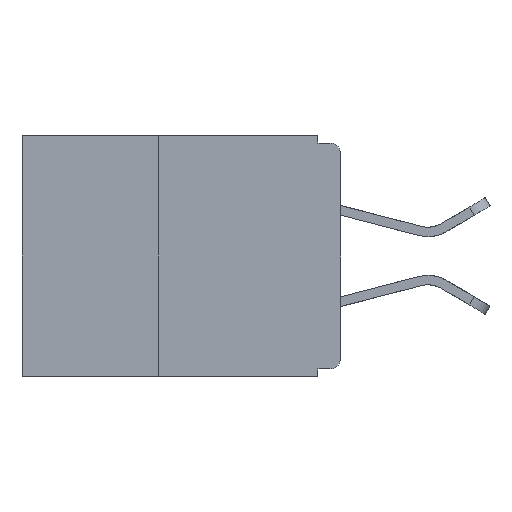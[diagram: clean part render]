
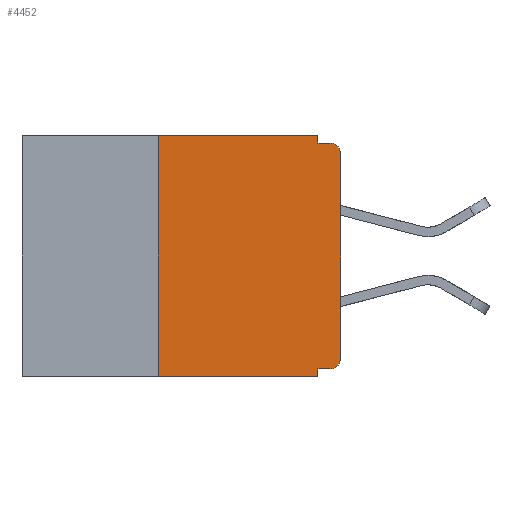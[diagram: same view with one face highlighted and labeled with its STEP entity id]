
A CAD part, left-side view. The second image highlights one B-rep face of the part: STEP entity #4452.
In plain terms, the highlighted planar face has unit normal (-1, 0, 0).
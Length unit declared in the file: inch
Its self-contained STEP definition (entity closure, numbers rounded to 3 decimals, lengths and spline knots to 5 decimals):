
#383 = DIRECTION ( 'NONE',  ( 1., 0., 0. ) ) ;
#982 = VECTOR ( 'NONE', #26300, 39.37008 ) ;
#1465 = CARTESIAN_POINT ( 'NONE',  ( 0., 0.437, 0. ) ) ;
#1678 = DIRECTION ( 'NONE',  ( 0., -1., 0. ) ) ;
#1950 = EDGE_CURVE ( 'NONE', #2396, #4100, #3413, .T. ) ;
#2301 = AXIS2_PLACEMENT_3D ( 'NONE', #21754, #9430, #23759 ) ;
#2396 = VERTEX_POINT ( 'NONE', #19117 ) ;
#2448 = CARTESIAN_POINT ( 'NONE',  ( 0., 0., -0.305 ) ) ;
#2530 = EDGE_CURVE ( 'NONE', #22444, #8970, #4804, .T. ) ;
#2553 = VERTEX_POINT ( 'NONE', #17504 ) ;
#2734 = CIRCLE ( 'NONE', #2301, 0.015 ) ;
#3050 = LINE ( 'NONE', #20234, #24468 ) ;
#3413 = CIRCLE ( 'NONE', #8752, 0.015 ) ;
#3708 = CARTESIAN_POINT ( 'NONE',  ( 0., 0.031, 0. ) ) ;
#3737 = PLANE ( 'NONE',  #25244 ) ;
#4100 = VERTEX_POINT ( 'NONE', #2448 ) ;
#4102 = LINE ( 'NONE', #18212, #24798 ) ;
#4452 = ADVANCED_FACE ( 'NONE', ( #10992 ), #3737, .F. ) ;
#4738 = VERTEX_POINT ( 'NONE', #19252 ) ;
#4804 = LINE ( 'NONE', #23291, #26603 ) ;
#5505 = LINE ( 'NONE', #3708, #982 ) ;
#6518 = EDGE_LOOP ( 'NONE', ( #24944, #15707, #7336, #26795, #16690, #24692, #26498, #8674, #20303, #11308 ) ) ;
#7336 = ORIENTED_EDGE ( 'NONE', *, *, #2530, .F. ) ;
#8523 = DIRECTION ( 'NONE',  ( 0., -1., 0. ) ) ;
#8674 = ORIENTED_EDGE ( 'NONE', *, *, #22145, .F. ) ;
#8752 = AXIS2_PLACEMENT_3D ( 'NONE', #15253, #18002, #26959 ) ;
#8970 = VERTEX_POINT ( 'NONE', #23158 ) ;
#9430 = DIRECTION ( 'NONE',  ( -1., 0., 0. ) ) ;
#10110 = DIRECTION ( 'NONE',  ( 0., 0., 1. ) ) ;
#10992 = FACE_OUTER_BOUND ( 'NONE', #6518, .T. ) ;
#11157 = EDGE_CURVE ( 'NONE', #4738, #22444, #5505, .T. ) ;
#11308 = ORIENTED_EDGE ( 'NONE', *, *, #1950, .T. ) ;
#11606 = LINE ( 'NONE', #24919, #21892 ) ;
#11624 = EDGE_CURVE ( 'NONE', #4100, #22159, #4102, .T. ) ;
#12183 = DIRECTION ( 'NONE',  ( 0., 1., 0. ) ) ;
#12957 = CARTESIAN_POINT ( 'NONE',  ( 0., 0.437, 0. ) ) ;
#14311 = CARTESIAN_POINT ( 'NONE',  ( 0., 0.25, 0. ) ) ;
#14985 = DIRECTION ( 'NONE',  ( 0., -1., 0. ) ) ;
#15226 = CARTESIAN_POINT ( 'NONE',  ( 0., 0.031, -0.01 ) ) ;
#15237 = EDGE_CURVE ( 'NONE', #19847, #19323, #3050, .T. ) ;
#15253 = CARTESIAN_POINT ( 'NONE',  ( 0., 0.015, -0.305 ) ) ;
#15657 = LINE ( 'NONE', #24407, #22442 ) ;
#15707 = ORIENTED_EDGE ( 'NONE', *, *, #24796, .T. ) ;
#16602 = EDGE_CURVE ( 'NONE', #19847, #25715, #11606, .T. ) ;
#16690 = ORIENTED_EDGE ( 'NONE', *, *, #21731, .F. ) ;
#17324 = LINE ( 'NONE', #12957, #22165 ) ;
#17504 = CARTESIAN_POINT ( 'NONE',  ( 0., 0.031, -0.32 ) ) ;
#17932 = EDGE_CURVE ( 'NONE', #2396, #2553, #15657, .T. ) ;
#18002 = DIRECTION ( 'NONE',  ( -1., 0., 0. ) ) ;
#18177 = DIRECTION ( 'NONE',  ( 0., 0., 1. ) ) ;
#18212 = CARTESIAN_POINT ( 'NONE',  ( 0., 0., 0. ) ) ;
#19117 = CARTESIAN_POINT ( 'NONE',  ( 0., 0.015, -0.32 ) ) ;
#19252 = CARTESIAN_POINT ( 'NONE',  ( 0., 0.031, 0. ) ) ;
#19323 = VERTEX_POINT ( 'NONE', #14311 ) ;
#19847 = VERTEX_POINT ( 'NONE', #26520 ) ;
#20234 = CARTESIAN_POINT ( 'NONE',  ( 0., 0.25, -0.33 ) ) ;
#20303 = ORIENTED_EDGE ( 'NONE', *, *, #17932, .F. ) ;
#20421 = CARTESIAN_POINT ( 'NONE',  ( 0., 0., -0.025 ) ) ;
#21528 = VECTOR ( 'NONE', #22455, 39.37008 ) ;
#21731 = EDGE_CURVE ( 'NONE', #19323, #4738, #17324, .T. ) ;
#21754 = CARTESIAN_POINT ( 'NONE',  ( 0., 0.015, -0.025 ) ) ;
#21892 = VECTOR ( 'NONE', #8523, 39.37008 ) ;
#22145 = EDGE_CURVE ( 'NONE', #2553, #25715, #26753, .T. ) ;
#22159 = VERTEX_POINT ( 'NONE', #20421 ) ;
#22165 = VECTOR ( 'NONE', #14985, 39.37008 ) ;
#22442 = VECTOR ( 'NONE', #12183, 39.37008 ) ;
#22444 = VERTEX_POINT ( 'NONE', #15226 ) ;
#22455 = DIRECTION ( 'NONE',  ( 0., 0., -1. ) ) ;
#23158 = CARTESIAN_POINT ( 'NONE',  ( 0., 0.015, -0.01 ) ) ;
#23291 = CARTESIAN_POINT ( 'NONE',  ( 0., 0., -0.01 ) ) ;
#23759 = DIRECTION ( 'NONE',  ( 0., 0., -1. ) ) ;
#24407 = CARTESIAN_POINT ( 'NONE',  ( 0., 0., -0.32 ) ) ;
#24468 = VECTOR ( 'NONE', #18177, 39.37008 ) ;
#24692 = ORIENTED_EDGE ( 'NONE', *, *, #15237, .F. ) ;
#24796 = EDGE_CURVE ( 'NONE', #22159, #8970, #2734, .T. ) ;
#24798 = VECTOR ( 'NONE', #10110, 39.37008 ) ;
#24919 = CARTESIAN_POINT ( 'NONE',  ( 0., 0.437, -0.33 ) ) ;
#24944 = ORIENTED_EDGE ( 'NONE', *, *, #11624, .T. ) ;
#25244 = AXIS2_PLACEMENT_3D ( 'NONE', #1465, #383, #26925 ) ;
#25715 = VERTEX_POINT ( 'NONE', #26601 ) ;
#26300 = DIRECTION ( 'NONE',  ( 0., 0., -1. ) ) ;
#26313 = CARTESIAN_POINT ( 'NONE',  ( 0., 0.031, -0.33 ) ) ;
#26498 = ORIENTED_EDGE ( 'NONE', *, *, #16602, .T. ) ;
#26520 = CARTESIAN_POINT ( 'NONE',  ( 0., 0.25, -0.33 ) ) ;
#26601 = CARTESIAN_POINT ( 'NONE',  ( 0., 0.031, -0.33 ) ) ;
#26603 = VECTOR ( 'NONE', #1678, 39.37008 ) ;
#26753 = LINE ( 'NONE', #26313, #21528 ) ;
#26795 = ORIENTED_EDGE ( 'NONE', *, *, #11157, .F. ) ;
#26925 = DIRECTION ( 'NONE',  ( 0., 0., -1. ) ) ;
#26959 = DIRECTION ( 'NONE',  ( 0., 0., -1. ) ) ;
